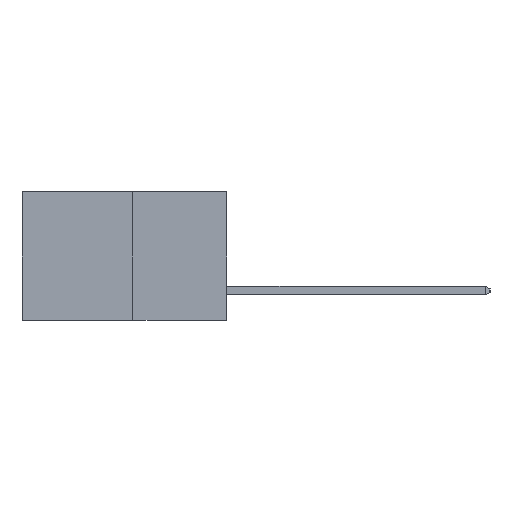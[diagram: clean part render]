
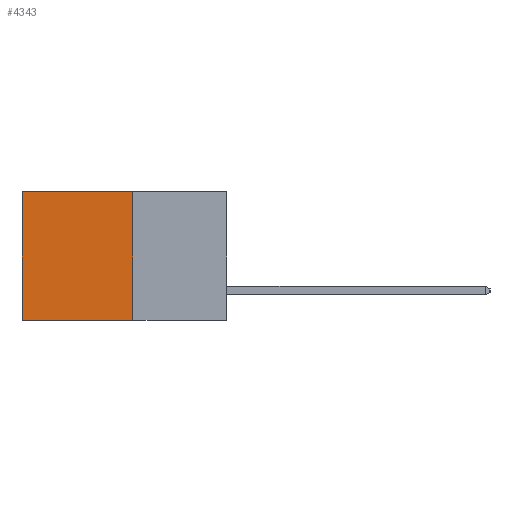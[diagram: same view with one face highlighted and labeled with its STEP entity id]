
A CAD part, left-side view. The second image highlights one B-rep face of the part: STEP entity #4343.
In plain terms, the highlighted planar face has unit normal (-1, 0, 0).
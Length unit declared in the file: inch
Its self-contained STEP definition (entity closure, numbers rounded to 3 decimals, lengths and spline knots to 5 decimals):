
#641 = EDGE_LOOP ( 'NONE', ( #5364, #6521, #3425, #2017 ) ) ;
#1174 = VECTOR ( 'NONE', #9379, 39.37008 ) ;
#1716 = EDGE_CURVE ( 'NONE', #6286, #12989, #15954, .T. ) ;
#2017 = ORIENTED_EDGE ( 'NONE', *, *, #14973, .T. ) ;
#2741 = LINE ( 'NONE', #8725, #18048 ) ;
#3037 = CARTESIAN_POINT ( 'NONE',  ( 0.277, 0.59, 0. ) ) ;
#3425 = ORIENTED_EDGE ( 'NONE', *, *, #9004, .F. ) ;
#4343 = ADVANCED_FACE ( 'NONE', ( #18549 ), #9798, .F. ) ;
#4902 = VERTEX_POINT ( 'NONE', #11883 ) ;
#5364 = ORIENTED_EDGE ( 'NONE', *, *, #1716, .T. ) ;
#5947 = CARTESIAN_POINT ( 'NONE',  ( 0.277, 0.27, -0.37 ) ) ;
#6286 = VERTEX_POINT ( 'NONE', #3037 ) ;
#6521 = ORIENTED_EDGE ( 'NONE', *, *, #15053, .F. ) ;
#8335 = CARTESIAN_POINT ( 'NONE',  ( 0.277, 0.59, -0.37 ) ) ;
#8725 = CARTESIAN_POINT ( 'NONE',  ( 0.277, 0.27, 0. ) ) ;
#9004 = EDGE_CURVE ( 'NONE', #15847, #4902, #16623, .T. ) ;
#9379 = DIRECTION ( 'NONE',  ( 0., 0., -1. ) ) ;
#9399 = DIRECTION ( 'NONE',  ( 0., 0., -1. ) ) ;
#9436 = DIRECTION ( 'NONE',  ( 1., 0., 0. ) ) ;
#9568 = CARTESIAN_POINT ( 'NONE',  ( 0.277, 0.27, -0.37 ) ) ;
#9798 = PLANE ( 'NONE',  #13677 ) ;
#11883 = CARTESIAN_POINT ( 'NONE',  ( 0.277, 0.27, -0.37 ) ) ;
#12125 = VECTOR ( 'NONE', #14464, 39.37008 ) ;
#12219 = CARTESIAN_POINT ( 'NONE',  ( 0.277, 0.27, -0.37 ) ) ;
#12448 = VECTOR ( 'NONE', #14581, 39.37008 ) ;
#12989 = VERTEX_POINT ( 'NONE', #8335 ) ;
#13677 = AXIS2_PLACEMENT_3D ( 'NONE', #9568, #9436, #9399 ) ;
#14464 = DIRECTION ( 'NONE',  ( 0., 0., -1. ) ) ;
#14581 = DIRECTION ( 'NONE',  ( 0., 1., 0. ) ) ;
#14973 = EDGE_CURVE ( 'NONE', #15847, #6286, #2741, .T. ) ;
#15053 = EDGE_CURVE ( 'NONE', #4902, #12989, #16712, .T. ) ;
#15099 = CARTESIAN_POINT ( 'NONE',  ( 0.277, 0.59, -0.37 ) ) ;
#15847 = VERTEX_POINT ( 'NONE', #17898 ) ;
#15954 = LINE ( 'NONE', #15099, #12125 ) ;
#16623 = LINE ( 'NONE', #12219, #1174 ) ;
#16712 = LINE ( 'NONE', #5947, #12448 ) ;
#17898 = CARTESIAN_POINT ( 'NONE',  ( 0.277, 0.27, 0. ) ) ;
#18048 = VECTOR ( 'NONE', #18698, 39.37008 ) ;
#18549 = FACE_OUTER_BOUND ( 'NONE', #641, .T. ) ;
#18698 = DIRECTION ( 'NONE',  ( 0., 1., 0. ) ) ;
